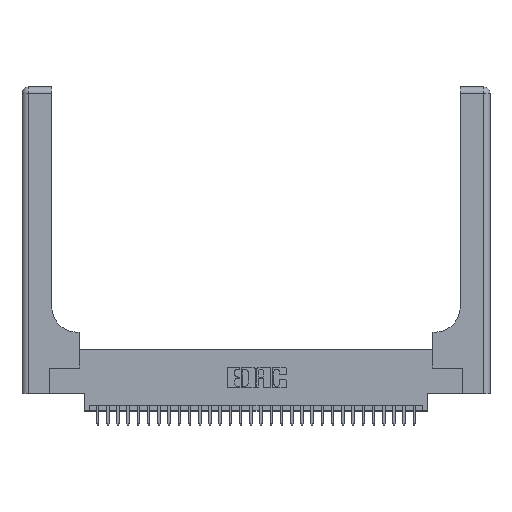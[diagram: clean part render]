
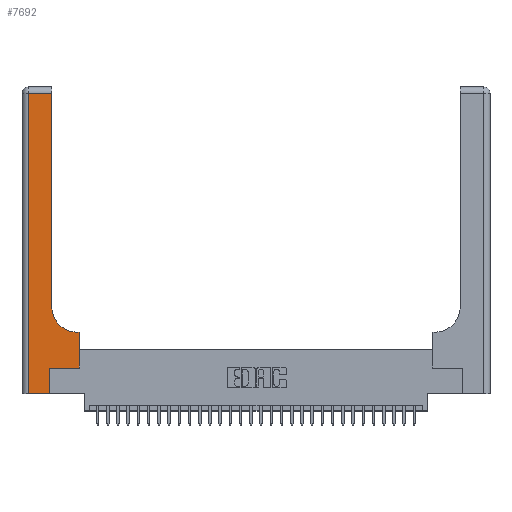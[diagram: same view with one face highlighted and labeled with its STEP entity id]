
A CAD part, top view. The second image highlights one B-rep face of the part: STEP entity #7692.
In plain terms, the highlighted planar face has unit normal (0, 0, 1).
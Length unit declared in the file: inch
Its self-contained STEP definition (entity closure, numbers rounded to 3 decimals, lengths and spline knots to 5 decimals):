
#840 = CARTESIAN_POINT ( 'NONE',  ( 0.06, 2.94, 0.37 ) ) ;
#1376 = CARTESIAN_POINT ( 'NONE',  ( 0.2915, 2.94, 0.37 ) ) ;
#1709 = VERTEX_POINT ( 'NONE', #25313 ) ;
#2221 = VERTEX_POINT ( 'NONE', #840 ) ;
#2287 = CARTESIAN_POINT ( 'NONE',  ( 0.5415, 0.85, 0.37 ) ) ;
#3598 = EDGE_CURVE ( 'NONE', #2221, #14312, #23599, .T. ) ;
#3798 = DIRECTION ( 'NONE',  ( 0., -1., 0. ) ) ;
#4176 = EDGE_CURVE ( 'NONE', #9324, #10047, #18918, .T. ) ;
#4338 = DIRECTION ( 'NONE',  ( 0., 1., 0. ) ) ;
#4698 = DIRECTION ( 'NONE',  ( -1., 0., 0. ) ) ;
#4712 = ORIENTED_EDGE ( 'NONE', *, *, #16537, .T. ) ;
#4885 = LINE ( 'NONE', #6974, #30244 ) ;
#5601 = EDGE_LOOP ( 'NONE', ( #22882, #7383, #13797, #6065, #25818, #25407, #15829, #19117, #4712 ) ) ;
#5936 = VECTOR ( 'NONE', #4698, 39.37008 ) ;
#6065 = ORIENTED_EDGE ( 'NONE', *, *, #26410, .T. ) ;
#6935 = CARTESIAN_POINT ( 'NONE',  ( 0., 2.94, 0.37 ) ) ;
#6974 = CARTESIAN_POINT ( 'NONE',  ( 0.2915, 3., 0.37 ) ) ;
#7006 = CARTESIAN_POINT ( 'NONE',  ( 0., 3., 0.37 ) ) ;
#7159 = LINE ( 'NONE', #24124, #7942 ) ;
#7195 = DIRECTION ( 'NONE',  ( 1., 0., 0. ) ) ;
#7383 = ORIENTED_EDGE ( 'NONE', *, *, #28904, .T. ) ;
#7515 = DIRECTION ( 'NONE',  ( 0., 0., -1. ) ) ;
#7692 = ADVANCED_FACE ( 'NONE', ( #29548 ), #9589, .F. ) ;
#7775 = CARTESIAN_POINT ( 'NONE',  ( 0.06, 3., 0.37 ) ) ;
#7942 = VECTOR ( 'NONE', #31692, 39.37008 ) ;
#9324 = VERTEX_POINT ( 'NONE', #16452 ) ;
#9445 = CARTESIAN_POINT ( 'NONE',  ( 0.5585, 0.6, 0.37 ) ) ;
#9589 = PLANE ( 'NONE',  #24365 ) ;
#9776 = CARTESIAN_POINT ( 'NONE',  ( 0.5585, 0.25, 0.37 ) ) ;
#10047 = VERTEX_POINT ( 'NONE', #19494 ) ;
#10544 = VERTEX_POINT ( 'NONE', #28225 ) ;
#11390 = VERTEX_POINT ( 'NONE', #12307 ) ;
#11910 = DIRECTION ( 'NONE',  ( 0., 1., 0. ) ) ;
#12307 = CARTESIAN_POINT ( 'NONE',  ( 0.5415, 0.6, 0.37 ) ) ;
#12472 = VERTEX_POINT ( 'NONE', #1376 ) ;
#12617 = LINE ( 'NONE', #9776, #29522 ) ;
#13797 = ORIENTED_EDGE ( 'NONE', *, *, #3598, .T. ) ;
#14014 = LINE ( 'NONE', #22279, #29814 ) ;
#14312 = VERTEX_POINT ( 'NONE', #27832 ) ;
#15829 = ORIENTED_EDGE ( 'NONE', *, *, #25828, .T. ) ;
#16452 = CARTESIAN_POINT ( 'NONE',  ( 0.269, 0., 0.37 ) ) ;
#16537 = EDGE_CURVE ( 'NONE', #11390, #1709, #24751, .T. ) ;
#17444 = VECTOR ( 'NONE', #3798, 39.37008 ) ;
#18918 = LINE ( 'NONE', #21387, #30139 ) ;
#19117 = ORIENTED_EDGE ( 'NONE', *, *, #28326, .T. ) ;
#19494 = CARTESIAN_POINT ( 'NONE',  ( 0.269, 0.25, 0.37 ) ) ;
#19546 = DIRECTION ( 'NONE',  ( 1., 0., 0. ) ) ;
#21387 = CARTESIAN_POINT ( 'NONE',  ( 0.269, 0., 0.37 ) ) ;
#21879 = DIRECTION ( 'NONE',  ( 0., 1., 0. ) ) ;
#22279 = CARTESIAN_POINT ( 'NONE',  ( 0.2915, 0.6, 0.37 ) ) ;
#22373 = CARTESIAN_POINT ( 'NONE',  ( 0., 0., 0.37 ) ) ;
#22882 = ORIENTED_EDGE ( 'NONE', *, *, #27664, .T. ) ;
#23371 = LINE ( 'NONE', #22373, #25626 ) ;
#23599 = LINE ( 'NONE', #7775, #17444 ) ;
#24124 = CARTESIAN_POINT ( 'NONE',  ( 0.269, 0.25, 0.37 ) ) ;
#24163 = DIRECTION ( 'NONE',  ( -1., 0., 0. ) ) ;
#24361 = EDGE_CURVE ( 'NONE', #10047, #10544, #7159, .T. ) ;
#24365 = AXIS2_PLACEMENT_3D ( 'NONE', #7006, #26646, #24163 ) ;
#24751 = CIRCLE ( 'NONE', #27698, 0.25 ) ;
#25313 = CARTESIAN_POINT ( 'NONE',  ( 0.2915, 0.85, 0.37 ) ) ;
#25407 = ORIENTED_EDGE ( 'NONE', *, *, #24361, .T. ) ;
#25626 = VECTOR ( 'NONE', #19546, 39.37008 ) ;
#25818 = ORIENTED_EDGE ( 'NONE', *, *, #4176, .T. ) ;
#25828 = EDGE_CURVE ( 'NONE', #10544, #27622, #12617, .T. ) ;
#26410 = EDGE_CURVE ( 'NONE', #14312, #9324, #23371, .T. ) ;
#26646 = DIRECTION ( 'NONE',  ( 0., 0., -1. ) ) ;
#27226 = DIRECTION ( 'NONE',  ( -1., 0., 0. ) ) ;
#27622 = VERTEX_POINT ( 'NONE', #9445 ) ;
#27664 = EDGE_CURVE ( 'NONE', #1709, #12472, #4885, .T. ) ;
#27698 = AXIS2_PLACEMENT_3D ( 'NONE', #2287, #7515, #7195 ) ;
#27832 = CARTESIAN_POINT ( 'NONE',  ( 0.06, 0., 0.37 ) ) ;
#28225 = CARTESIAN_POINT ( 'NONE',  ( 0.5585, 0.25, 0.37 ) ) ;
#28326 = EDGE_CURVE ( 'NONE', #27622, #11390, #14014, .T. ) ;
#28904 = EDGE_CURVE ( 'NONE', #12472, #2221, #29371, .T. ) ;
#29371 = LINE ( 'NONE', #6935, #5936 ) ;
#29522 = VECTOR ( 'NONE', #11910, 39.37008 ) ;
#29548 = FACE_OUTER_BOUND ( 'NONE', #5601, .T. ) ;
#29814 = VECTOR ( 'NONE', #27226, 39.37008 ) ;
#30139 = VECTOR ( 'NONE', #4338, 39.37008 ) ;
#30244 = VECTOR ( 'NONE', #21879, 39.37008 ) ;
#31692 = DIRECTION ( 'NONE',  ( 1., 0., 0. ) ) ;
